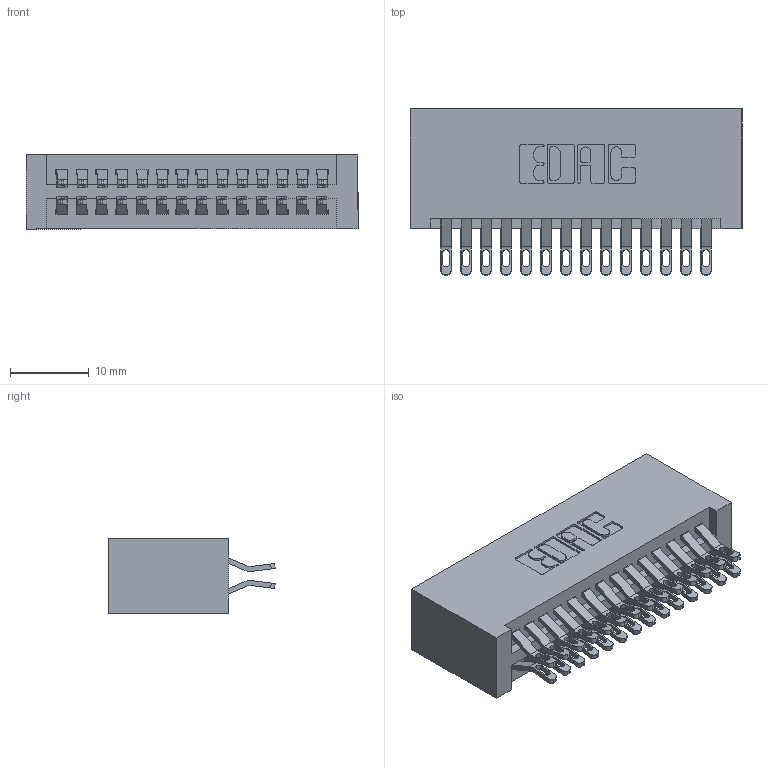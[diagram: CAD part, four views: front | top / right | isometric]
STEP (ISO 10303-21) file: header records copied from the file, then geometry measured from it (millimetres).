
FILE_DESCRIPTION (( 'STEP AP203' ), '1' );
FILE_NAME ('395-028-555-201.STEP', '2019-10-16T20:00:36', ( '' ), ( '' ), 'SwSTEP 2.0', 'SolidWorks 2016', '' );
FILE_SCHEMA (( 'CONFIG_CONTROL_DESIGN' ));
Length unit declared in the file: inch
Products named in the file (3): 345 Part_No Mounting Lugs; 345-292-001_555 Tail; 395-028-555-201
Assembly tree (29 placements, depth 2):
  395-028-555-201
    345 Part_No Mounting Lugs
    345-292-001_555 Tail  x28
Bounding box: 42.16 x 21.13 x 9.4 mm (x, y, z)
Volume: 4533.1 mm3; surface area: 6744.1 mm2
Topology: 29 solids, 29 shells, 1686 faces, 5273 edges, 3514 vertices
Faces by surface type: plane 944, cylinder 742
Entity records: 14803 total; most frequent: CARTESIAN_POINT 2542, ORIENTED_EDGE 2446, DIRECTION 2239, EDGE_CURVE 1223, VECTOR 1023, LINE 1023, VERTEX_POINT 814, AXIS2_PLACEMENT_3D 608
